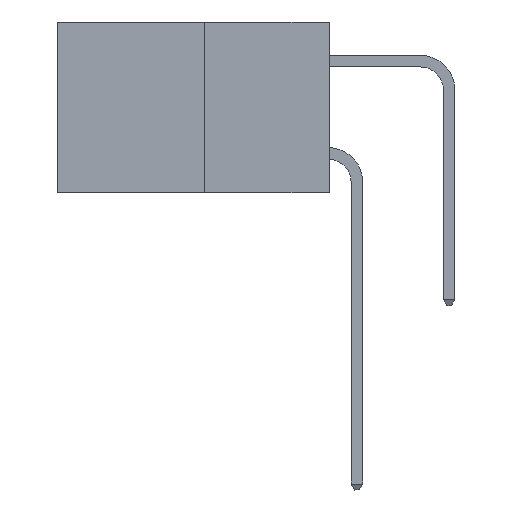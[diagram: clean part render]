
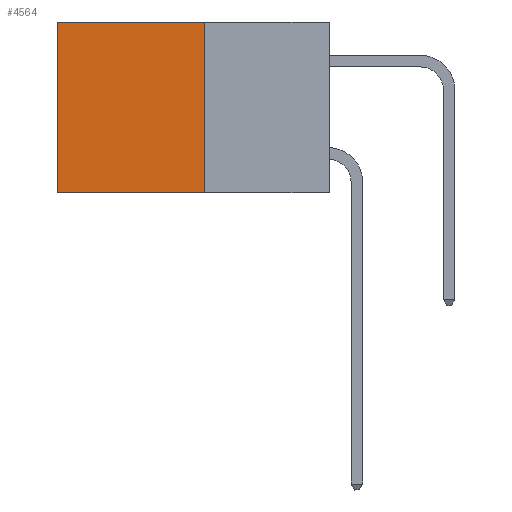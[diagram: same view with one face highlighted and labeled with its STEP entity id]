
A CAD part, left-side view. The second image highlights one B-rep face of the part: STEP entity #4564.
In plain terms, the highlighted planar face has unit normal (-1, 0, 0).
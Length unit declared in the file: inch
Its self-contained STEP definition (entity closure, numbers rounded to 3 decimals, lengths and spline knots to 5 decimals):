
#118 = CARTESIAN_POINT ( 'NONE',  ( 0.277, 0.27, -0.37 ) ) ;
#1355 = EDGE_CURVE ( 'NONE', #1801, #11296, #5173, .T. ) ;
#1801 = VERTEX_POINT ( 'NONE', #7075 ) ;
#2284 = VERTEX_POINT ( 'NONE', #3202 ) ;
#3202 = CARTESIAN_POINT ( 'NONE',  ( 0.277, 0.27, -0.37 ) ) ;
#3925 = FACE_OUTER_BOUND ( 'NONE', #7897, .T. ) ;
#3941 = CARTESIAN_POINT ( 'NONE',  ( 0.277, 0.59, -0.37 ) ) ;
#4327 = DIRECTION ( 'NONE',  ( 0., 0., -1. ) ) ;
#4413 = ORIENTED_EDGE ( 'NONE', *, *, #1355, .T. ) ;
#4426 = VECTOR ( 'NONE', #13041, 39.37008 ) ;
#4564 = ADVANCED_FACE ( 'NONE', ( #3925 ), #7047, .F. ) ;
#4774 = EDGE_CURVE ( 'NONE', #7670, #1801, #12503, .T. ) ;
#4794 = AXIS2_PLACEMENT_3D ( 'NONE', #7718, #6761, #6814 ) ;
#4844 = VECTOR ( 'NONE', #9932, 39.37008 ) ;
#5173 = LINE ( 'NONE', #3941, #4844 ) ;
#6162 = VECTOR ( 'NONE', #12894, 39.37008 ) ;
#6761 = DIRECTION ( 'NONE',  ( 1., 0., 0. ) ) ;
#6771 = ORIENTED_EDGE ( 'NONE', *, *, #12516, .F. ) ;
#6814 = DIRECTION ( 'NONE',  ( 0., 0., -1. ) ) ;
#6982 = ORIENTED_EDGE ( 'NONE', *, *, #12223, .F. ) ;
#7047 = PLANE ( 'NONE',  #4794 ) ;
#7075 = CARTESIAN_POINT ( 'NONE',  ( 0.277, 0.59, 0. ) ) ;
#7380 = ORIENTED_EDGE ( 'NONE', *, *, #4774, .T. ) ;
#7670 = VERTEX_POINT ( 'NONE', #10211 ) ;
#7718 = CARTESIAN_POINT ( 'NONE',  ( 0.277, 0.27, -0.37 ) ) ;
#7897 = EDGE_LOOP ( 'NONE', ( #4413, #6771, #6982, #7380 ) ) ;
#9422 = VECTOR ( 'NONE', #4327, 39.37008 ) ;
#9932 = DIRECTION ( 'NONE',  ( 0., 0., -1. ) ) ;
#10211 = CARTESIAN_POINT ( 'NONE',  ( 0.277, 0.27, 0. ) ) ;
#11296 = VERTEX_POINT ( 'NONE', #11824 ) ;
#11522 = LINE ( 'NONE', #11916, #6162 ) ;
#11824 = CARTESIAN_POINT ( 'NONE',  ( 0.277, 0.59, -0.37 ) ) ;
#11916 = CARTESIAN_POINT ( 'NONE',  ( 0.277, 0.27, -0.37 ) ) ;
#11949 = LINE ( 'NONE', #118, #9422 ) ;
#12223 = EDGE_CURVE ( 'NONE', #7670, #2284, #11949, .T. ) ;
#12503 = LINE ( 'NONE', #13022, #4426 ) ;
#12516 = EDGE_CURVE ( 'NONE', #2284, #11296, #11522, .T. ) ;
#12894 = DIRECTION ( 'NONE',  ( 0., 1., 0. ) ) ;
#13022 = CARTESIAN_POINT ( 'NONE',  ( 0.277, 0.27, 0. ) ) ;
#13041 = DIRECTION ( 'NONE',  ( 0., 1., 0. ) ) ;
